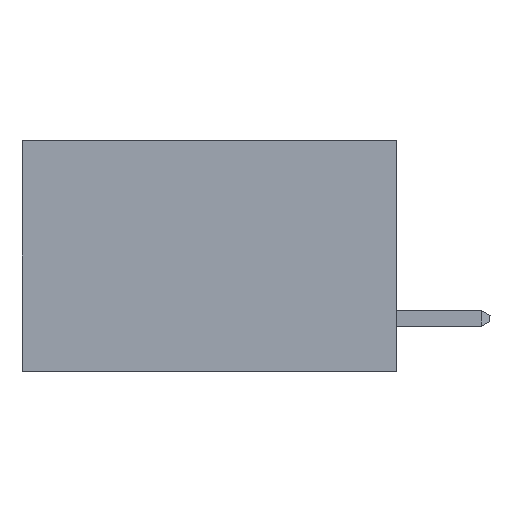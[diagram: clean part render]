
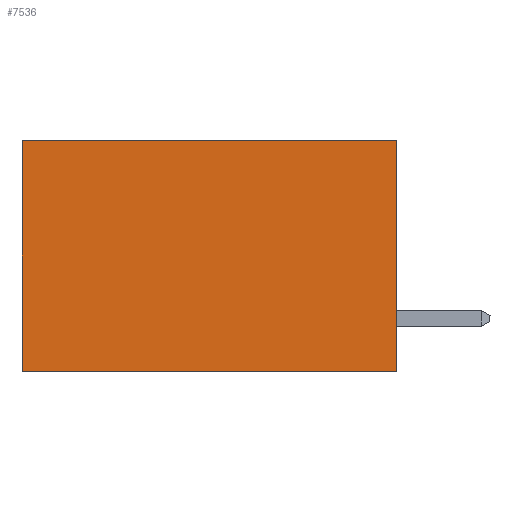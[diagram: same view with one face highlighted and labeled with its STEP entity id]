
A CAD part, left-side view. The second image highlights one B-rep face of the part: STEP entity #7536.
In plain terms, the highlighted planar face has unit normal (-1, 0, 0).
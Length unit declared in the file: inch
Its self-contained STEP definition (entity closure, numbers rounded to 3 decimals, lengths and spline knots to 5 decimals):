
#39 = ORIENTED_EDGE ( 'NONE', *, *, #2369, .T. ) ;
#133 = LINE ( 'NONE', #440, #250 ) ;
#228 = ORIENTED_EDGE ( 'NONE', *, *, #5420, .T. ) ;
#250 = VECTOR ( 'NONE', #317, 39.37008 ) ;
#317 = DIRECTION ( 'NONE',  ( 0., 1., 0. ) ) ;
#333 = LINE ( 'NONE', #2658, #5926 ) ;
#440 = CARTESIAN_POINT ( 'NONE',  ( 0.298, 0., 0. ) ) ;
#1061 = CARTESIAN_POINT ( 'NONE',  ( 0.298, 0., -0.37 ) ) ;
#1979 = CARTESIAN_POINT ( 'NONE',  ( 0.298, 0., 0. ) ) ;
#2357 = LINE ( 'NONE', #1979, #5439 ) ;
#2369 = EDGE_CURVE ( 'NONE', #9408, #6523, #333, .T. ) ;
#2407 = EDGE_LOOP ( 'NONE', ( #39, #2517, #9005, #228 ) ) ;
#2491 = AXIS2_PLACEMENT_3D ( 'NONE', #2667, #4119, #4025 ) ;
#2517 = ORIENTED_EDGE ( 'NONE', *, *, #9411, .F. ) ;
#2563 = VECTOR ( 'NONE', #5402, 39.37008 ) ;
#2582 = CARTESIAN_POINT ( 'NONE',  ( 0.298, 0.6, 0. ) ) ;
#2658 = CARTESIAN_POINT ( 'NONE',  ( 0.298, 0.6, 0. ) ) ;
#2667 = CARTESIAN_POINT ( 'NONE',  ( 0.298, 0., 0. ) ) ;
#2690 = DIRECTION ( 'NONE',  ( 0., 0., -1. ) ) ;
#2996 = VERTEX_POINT ( 'NONE', #8375 ) ;
#3291 = EDGE_CURVE ( 'NONE', #2996, #6477, #2357, .T. ) ;
#4025 = DIRECTION ( 'NONE',  ( 0., 0., -1. ) ) ;
#4119 = DIRECTION ( 'NONE',  ( 1., 0., 0. ) ) ;
#5165 = LINE ( 'NONE', #8419, #2563 ) ;
#5402 = DIRECTION ( 'NONE',  ( 0., 1., 0. ) ) ;
#5420 = EDGE_CURVE ( 'NONE', #2996, #9408, #133, .T. ) ;
#5439 = VECTOR ( 'NONE', #2690, 39.37008 ) ;
#5926 = VECTOR ( 'NONE', #9340, 39.37008 ) ;
#6477 = VERTEX_POINT ( 'NONE', #1061 ) ;
#6523 = VERTEX_POINT ( 'NONE', #6960 ) ;
#6960 = CARTESIAN_POINT ( 'NONE',  ( 0.298, 0.6, -0.37 ) ) ;
#7173 = FACE_OUTER_BOUND ( 'NONE', #2407, .T. ) ;
#7536 = ADVANCED_FACE ( 'NONE', ( #7173 ), #8500, .F. ) ;
#8375 = CARTESIAN_POINT ( 'NONE',  ( 0.298, 0., 0. ) ) ;
#8419 = CARTESIAN_POINT ( 'NONE',  ( 0.298, 0., -0.37 ) ) ;
#8500 = PLANE ( 'NONE',  #2491 ) ;
#9005 = ORIENTED_EDGE ( 'NONE', *, *, #3291, .F. ) ;
#9340 = DIRECTION ( 'NONE',  ( 0., 0., -1. ) ) ;
#9408 = VERTEX_POINT ( 'NONE', #2582 ) ;
#9411 = EDGE_CURVE ( 'NONE', #6477, #6523, #5165, .T. ) ;
